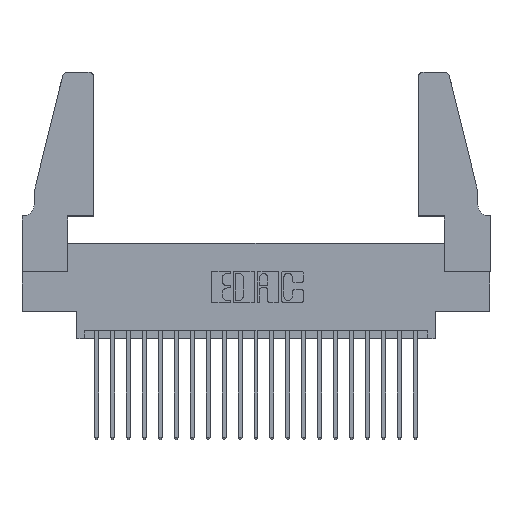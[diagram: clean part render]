
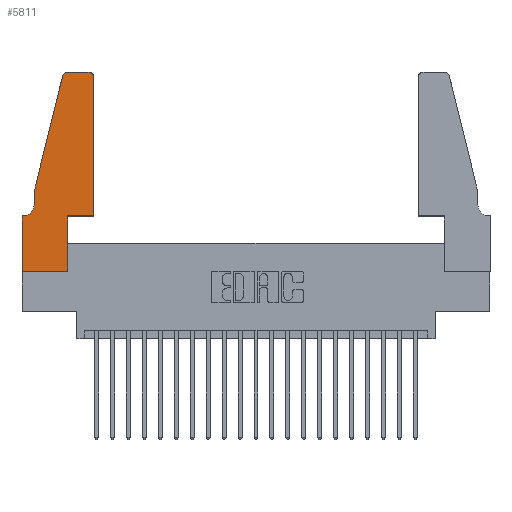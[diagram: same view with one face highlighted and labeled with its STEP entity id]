
A CAD part, top view. The second image highlights one B-rep face of the part: STEP entity #5811.
In plain terms, the highlighted planar face has unit normal (0, 0, 1).
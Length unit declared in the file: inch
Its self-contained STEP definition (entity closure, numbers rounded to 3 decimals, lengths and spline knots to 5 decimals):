
#663 = CARTESIAN_POINT ( 'NONE',  ( 0., 0., 0.37 ) ) ;
#749 = CIRCLE ( 'NONE', #6115, 0.03 ) ;
#1046 = ORIENTED_EDGE ( 'NONE', *, *, #10685, .T. ) ;
#1307 = DIRECTION ( 'NONE',  ( 0., 1., 0. ) ) ;
#1468 = VECTOR ( 'NONE', #15753, 39.37008 ) ;
#1472 = VECTOR ( 'NONE', #20731, 39.37008 ) ;
#1751 = EDGE_CURVE ( 'NONE', #7588, #6066, #18287, .T. ) ;
#2482 = LINE ( 'NONE', #13597, #7016 ) ;
#2950 = VECTOR ( 'NONE', #3495, 39.37008 ) ;
#3021 = CARTESIAN_POINT ( 'NONE',  ( 0.4505, 1.22, 0.37 ) ) ;
#3403 = VERTEX_POINT ( 'NONE', #7306 ) ;
#3495 = DIRECTION ( 'NONE',  ( -1., 0., 0. ) ) ;
#3528 = DIRECTION ( 'NONE',  ( 1., 0., 0. ) ) ;
#3681 = EDGE_CURVE ( 'NONE', #9342, #11075, #15603, .T. ) ;
#4026 = EDGE_CURVE ( 'NONE', #18383, #4407, #13819, .T. ) ;
#4388 = ORIENTED_EDGE ( 'NONE', *, *, #4026, .T. ) ;
#4407 = VERTEX_POINT ( 'NONE', #10109 ) ;
#4700 = DIRECTION ( 'NONE',  ( 0., 1., 0. ) ) ;
#5114 = ORIENTED_EDGE ( 'NONE', *, *, #5672, .T. ) ;
#5468 = CARTESIAN_POINT ( 'NONE',  ( 0.284, 1.22, 0.37 ) ) ;
#5672 = EDGE_CURVE ( 'NONE', #11075, #8900, #20562, .T. ) ;
#5811 = ADVANCED_FACE ( 'NONE', ( #21299 ), #11938, .T. ) ;
#6021 = CARTESIAN_POINT ( 'NONE',  ( 0., 0.35, 0.37 ) ) ;
#6066 = VERTEX_POINT ( 'NONE', #12499 ) ;
#6082 = LINE ( 'NONE', #663, #1472 ) ;
#6115 = AXIS2_PLACEMENT_3D ( 'NONE', #5468, #17069, #7169 ) ;
#6289 = CARTESIAN_POINT ( 'NONE',  ( 0.2865, 0.35, 0.37 ) ) ;
#6472 = VERTEX_POINT ( 'NONE', #14592 ) ;
#6547 = CARTESIAN_POINT ( 'NONE',  ( 0.4205, 1.22, 0.37 ) ) ;
#7016 = VECTOR ( 'NONE', #10323, 39.37008 ) ;
#7169 = DIRECTION ( 'NONE',  ( 1., 0., 0. ) ) ;
#7277 = CARTESIAN_POINT ( 'NONE',  ( 0.0055, 0.42, 0.37 ) ) ;
#7306 = CARTESIAN_POINT ( 'NONE',  ( 0.284, 1.25, 0.37 ) ) ;
#7568 = ORIENTED_EDGE ( 'NONE', *, *, #15154, .T. ) ;
#7588 = VERTEX_POINT ( 'NONE', #6021 ) ;
#7930 = VECTOR ( 'NONE', #19754, 39.37008 ) ;
#7934 = AXIS2_PLACEMENT_3D ( 'NONE', #6547, #18109, #8293 ) ;
#8293 = DIRECTION ( 'NONE',  ( 1., 0., 0. ) ) ;
#8397 = VERTEX_POINT ( 'NONE', #6289 ) ;
#8503 = CARTESIAN_POINT ( 'NONE',  ( 0.2865, 0., 0.37 ) ) ;
#8802 = ORIENTED_EDGE ( 'NONE', *, *, #3681, .T. ) ;
#8900 = VERTEX_POINT ( 'NONE', #17491 ) ;
#9013 = DIRECTION ( 'NONE',  ( -1., 0., 0. ) ) ;
#9342 = VERTEX_POINT ( 'NONE', #18676 ) ;
#9438 = EDGE_CURVE ( 'NONE', #8397, #9342, #19915, .T. ) ;
#10077 = CARTESIAN_POINT ( 'NONE',  ( 0.0755, 0.42, 0.37 ) ) ;
#10109 = CARTESIAN_POINT ( 'NONE',  ( 0.0055, 0.35, 0.37 ) ) ;
#10196 = VERTEX_POINT ( 'NONE', #19053 ) ;
#10323 = DIRECTION ( 'NONE',  ( -1., 0., 0. ) ) ;
#10525 = ORIENTED_EDGE ( 'NONE', *, *, #15185, .T. ) ;
#10592 = EDGE_CURVE ( 'NONE', #8900, #3403, #2482, .T. ) ;
#10603 = LINE ( 'NONE', #20547, #1468 ) ;
#10670 = ORIENTED_EDGE ( 'NONE', *, *, #1751, .T. ) ;
#10685 = EDGE_CURVE ( 'NONE', #3403, #6472, #749, .T. ) ;
#10795 = CARTESIAN_POINT ( 'NONE',  ( 0.4505, 0.35, 0.37 ) ) ;
#11075 = VERTEX_POINT ( 'NONE', #3021 ) ;
#11309 = VECTOR ( 'NONE', #4700, 39.37008 ) ;
#11432 = ORIENTED_EDGE ( 'NONE', *, *, #13429, .T. ) ;
#11902 = CARTESIAN_POINT ( 'NONE',  ( 0.0755, 0.35, 0.37 ) ) ;
#11938 = PLANE ( 'NONE',  #18917 ) ;
#12153 = CARTESIAN_POINT ( 'NONE',  ( 0., 0., 0.37 ) ) ;
#12499 = CARTESIAN_POINT ( 'NONE',  ( 0., 0., 0.37 ) ) ;
#12796 = VERTEX_POINT ( 'NONE', #8503 ) ;
#13074 = CARTESIAN_POINT ( 'NONE',  ( 0.4505, 0.35, 0.37 ) ) ;
#13429 = EDGE_CURVE ( 'NONE', #4407, #7588, #16739, .T. ) ;
#13561 = DIRECTION ( 'NONE',  ( 0., 0., 1. ) ) ;
#13597 = CARTESIAN_POINT ( 'NONE',  ( 0.2605, 1.25, 0.37 ) ) ;
#13819 = CIRCLE ( 'NONE', #17688, 0.07 ) ;
#14149 = ORIENTED_EDGE ( 'NONE', *, *, #16858, .T. ) ;
#14466 = VECTOR ( 'NONE', #14495, 39.37008 ) ;
#14495 = DIRECTION ( 'NONE',  ( 0., -1., 0. ) ) ;
#14592 = CARTESIAN_POINT ( 'NONE',  ( 0.25487, 1.22718, 0.37 ) ) ;
#15154 = EDGE_CURVE ( 'NONE', #12796, #8397, #20935, .T. ) ;
#15185 = EDGE_CURVE ( 'NONE', #10196, #18383, #15637, .T. ) ;
#15603 = LINE ( 'NONE', #13074, #11309 ) ;
#15609 = VECTOR ( 'NONE', #20469, 39.37008 ) ;
#15637 = LINE ( 'NONE', #16502, #7930 ) ;
#15753 = DIRECTION ( 'NONE',  ( -0.239, -0.971, 0. ) ) ;
#16145 = EDGE_CURVE ( 'NONE', #6472, #10196, #10603, .T. ) ;
#16502 = CARTESIAN_POINT ( 'NONE',  ( 0.0755, 0.5, 0.37 ) ) ;
#16739 = LINE ( 'NONE', #11902, #2950 ) ;
#16858 = EDGE_CURVE ( 'NONE', #6066, #12796, #6082, .T. ) ;
#17045 = ORIENTED_EDGE ( 'NONE', *, *, #10592, .T. ) ;
#17069 = DIRECTION ( 'NONE',  ( 0., 0., 1. ) ) ;
#17491 = CARTESIAN_POINT ( 'NONE',  ( 0.4205, 1.25, 0.37 ) ) ;
#17688 = AXIS2_PLACEMENT_3D ( 'NONE', #7277, #18789, #9013 ) ;
#17701 = EDGE_LOOP ( 'NONE', ( #17045, #1046, #19159, #10525, #4388, #11432, #10670, #14149, #7568, #20353, #8802, #5114 ) ) ;
#18109 = DIRECTION ( 'NONE',  ( 0., 0., 1. ) ) ;
#18287 = LINE ( 'NONE', #12153, #14466 ) ;
#18383 = VERTEX_POINT ( 'NONE', #10077 ) ;
#18676 = CARTESIAN_POINT ( 'NONE',  ( 0.4505, 0.35, 0.37 ) ) ;
#18789 = DIRECTION ( 'NONE',  ( 0., 0., -1. ) ) ;
#18917 = AXIS2_PLACEMENT_3D ( 'NONE', #21579, #13561, #3528 ) ;
#19053 = CARTESIAN_POINT ( 'NONE',  ( 0.0755, 0.5, 0.37 ) ) ;
#19159 = ORIENTED_EDGE ( 'NONE', *, *, #16145, .T. ) ;
#19754 = DIRECTION ( 'NONE',  ( 0., -1., 0. ) ) ;
#19915 = LINE ( 'NONE', #10795, #15609 ) ;
#20353 = ORIENTED_EDGE ( 'NONE', *, *, #9438, .T. ) ;
#20469 = DIRECTION ( 'NONE',  ( 1., 0., 0. ) ) ;
#20547 = CARTESIAN_POINT ( 'NONE',  ( 0.0755, 0.5, 0.37 ) ) ;
#20562 = CIRCLE ( 'NONE', #7934, 0.03 ) ;
#20731 = DIRECTION ( 'NONE',  ( 1., 0., 0. ) ) ;
#20935 = LINE ( 'NONE', #21211, #21429 ) ;
#21211 = CARTESIAN_POINT ( 'NONE',  ( 0.2865, 0.35, 0.37 ) ) ;
#21299 = FACE_OUTER_BOUND ( 'NONE', #17701, .T. ) ;
#21429 = VECTOR ( 'NONE', #1307, 39.37008 ) ;
#21579 = CARTESIAN_POINT ( 'NONE',  ( 0., 0.35, 0.37 ) ) ;
